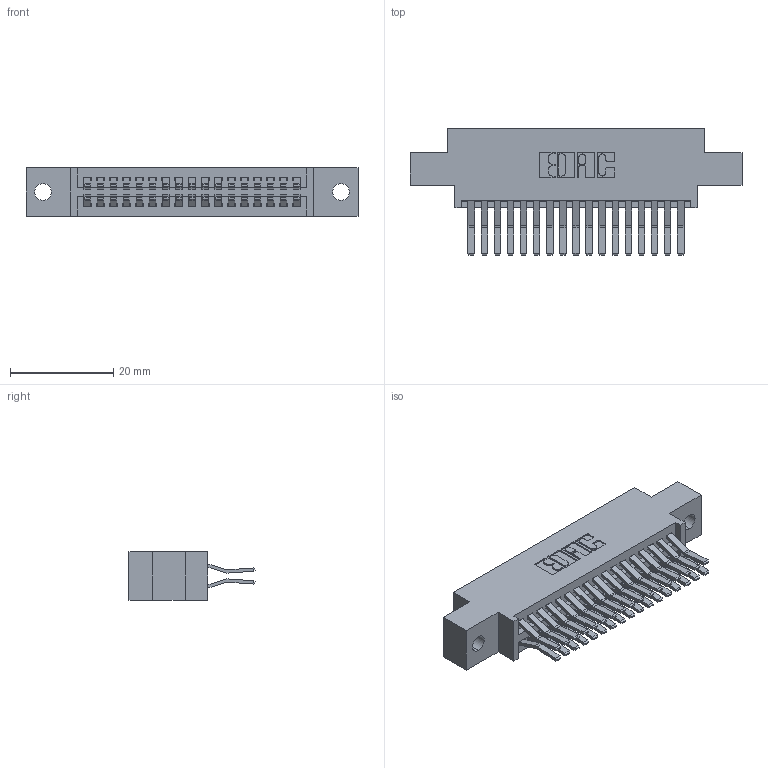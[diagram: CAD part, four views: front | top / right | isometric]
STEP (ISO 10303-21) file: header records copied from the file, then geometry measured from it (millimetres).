
FILE_DESCRIPTION (( 'STEP AP203' ), '1' );
FILE_NAME ('345-034-560-802.STEP', '2019-10-28T11:01:33', ( '' ), ( '' ), 'SwSTEP 2.0', 'SolidWorks 2016', '' );
FILE_SCHEMA (( 'CONFIG_CONTROL_DESIGN' ));
Length unit declared in the file: inch
Products named in the file (3): 345 Part_0.170 Offset - 0.128 Dia; 345-034-560-802; 345-292-001_560 Tail
Assembly tree (35 placements, depth 2):
  345-034-560-802
    345 Part_0.170 Offset - 0.128 Dia
    345-292-001_560 Tail  x34
Bounding box: 64.39 x 24.45 x 9.4 mm (x, y, z)
Volume: 6095.5 mm3; surface area: 8970 mm2
Topology: 35 solids, 35 shells, 1898 faces, 5623 edges, 3702 vertices
Faces by surface type: plane 1206, cylinder 692
Entity records: 16927 total; most frequent: CARTESIAN_POINT 2864, ORIENTED_EDGE 2798, DIRECTION 2559, EDGE_CURVE 1399, LINE 1195, VECTOR 1195, VERTEX_POINT 930, AXIS2_PLACEMENT_3D 682
